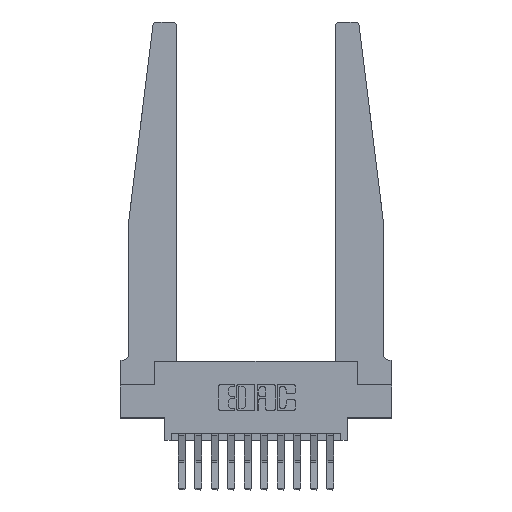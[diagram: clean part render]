
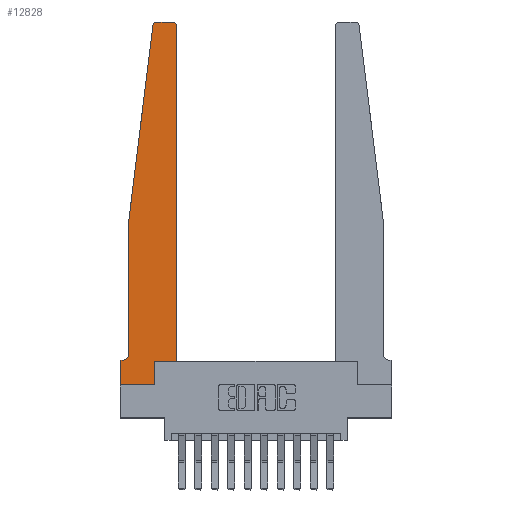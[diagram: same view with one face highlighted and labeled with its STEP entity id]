
A CAD part, top view. The second image highlights one B-rep face of the part: STEP entity #12828.
In plain terms, the highlighted planar face has unit normal (0, 0, 1).
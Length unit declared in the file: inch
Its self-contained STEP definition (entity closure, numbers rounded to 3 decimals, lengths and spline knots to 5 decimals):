
#224 = DIRECTION ( 'NONE',  ( 0., -1., 0. ) ) ;
#311 = VECTOR ( 'NONE', #13457, 39.37008 ) ;
#659 = DIRECTION ( 'NONE',  ( 1., 0., 0. ) ) ;
#852 = EDGE_LOOP ( 'NONE', ( #8478, #11043, #6783, #9050, #4390, #16160, #5548, #2327, #15677, #2943, #4963, #11494 ) ) ;
#966 = VERTEX_POINT ( 'NONE', #7093 ) ;
#1336 = DIRECTION ( 'NONE',  ( 0., 0., 1. ) ) ;
#1427 = CARTESIAN_POINT ( 'NONE',  ( 0., 0.1875, 0.37 ) ) ;
#1507 = EDGE_CURVE ( 'NONE', #2452, #4748, #9371, .T. ) ;
#1512 = VERTEX_POINT ( 'NONE', #13615 ) ;
#1540 = CARTESIAN_POINT ( 'NONE',  ( 0., 0., 0.37 ) ) ;
#1623 = AXIS2_PLACEMENT_3D ( 'NONE', #6373, #7605, #7774 ) ;
#1790 = CARTESIAN_POINT ( 'NONE',  ( 0.27653, 2.72, 0.37 ) ) ;
#2063 = VERTEX_POINT ( 'NONE', #3731 ) ;
#2226 = AXIS2_PLACEMENT_3D ( 'NONE', #1427, #1336, #9835 ) ;
#2267 = EDGE_CURVE ( 'NONE', #15915, #15272, #12274, .T. ) ;
#2270 = EDGE_CURVE ( 'NONE', #12565, #966, #16127, .T. ) ;
#2327 = ORIENTED_EDGE ( 'NONE', *, *, #6357, .T. ) ;
#2452 = VERTEX_POINT ( 'NONE', #2868 ) ;
#2659 = EDGE_CURVE ( 'NONE', #2063, #2452, #16177, .T. ) ;
#2868 = CARTESIAN_POINT ( 'NONE',  ( 0.2605, 0.18, 0.37 ) ) ;
#2943 = ORIENTED_EDGE ( 'NONE', *, *, #1507, .T. ) ;
#3179 = EDGE_CURVE ( 'NONE', #15272, #12565, #8724, .T. ) ;
#3459 = EDGE_CURVE ( 'NONE', #4748, #9136, #9968, .T. ) ;
#3561 = DIRECTION ( 'NONE',  ( 0., -1., 0. ) ) ;
#3731 = CARTESIAN_POINT ( 'NONE',  ( 0.2605, 0., 0.37 ) ) ;
#4014 = DIRECTION ( 'NONE',  ( -0.122, -0.992, 0. ) ) ;
#4219 = DIRECTION ( 'NONE',  ( -1., 0., 0. ) ) ;
#4390 = ORIENTED_EDGE ( 'NONE', *, *, #3179, .T. ) ;
#4739 = CARTESIAN_POINT ( 'NONE',  ( 0., 0., 0.37 ) ) ;
#4748 = VERTEX_POINT ( 'NONE', #13323 ) ;
#4963 = ORIENTED_EDGE ( 'NONE', *, *, #3459, .T. ) ;
#5191 = EDGE_CURVE ( 'NONE', #966, #12253, #5245, .T. ) ;
#5245 = LINE ( 'NONE', #11485, #8251 ) ;
#5548 = ORIENTED_EDGE ( 'NONE', *, *, #5191, .T. ) ;
#5680 = CIRCLE ( 'NONE', #14848, 0.03 ) ;
#5836 = DIRECTION ( 'NONE',  ( 0., 0., 1. ) ) ;
#6187 = CIRCLE ( 'NONE', #11174, 0.03 ) ;
#6225 = FACE_OUTER_BOUND ( 'NONE', #852, .T. ) ;
#6357 = EDGE_CURVE ( 'NONE', #12253, #2063, #11417, .T. ) ;
#6373 = CARTESIAN_POINT ( 'NONE',  ( 0.015, 0.2375, 0.37 ) ) ;
#6566 = DIRECTION ( 'NONE',  ( 1., 0., 0. ) ) ;
#6783 = ORIENTED_EDGE ( 'NONE', *, *, #9160, .T. ) ;
#6831 = DIRECTION ( 'NONE',  ( 0., 0., 1. ) ) ;
#7069 = CARTESIAN_POINT ( 'NONE',  ( 0.24675, 2.72367, 0.37 ) ) ;
#7093 = CARTESIAN_POINT ( 'NONE',  ( 0., 0.1875, 0.37 ) ) ;
#7200 = CARTESIAN_POINT ( 'NONE',  ( 0.065, 0.1875, 0.37 ) ) ;
#7348 = CARTESIAN_POINT ( 'NONE',  ( 0.065, 1.25, 0.37 ) ) ;
#7605 = DIRECTION ( 'NONE',  ( 0., 0., -1. ) ) ;
#7640 = EDGE_CURVE ( 'NONE', #9136, #1512, #5680, .T. ) ;
#7774 = DIRECTION ( 'NONE',  ( -1., 0., 0. ) ) ;
#8003 = VERTEX_POINT ( 'NONE', #7069 ) ;
#8140 = DIRECTION ( 'NONE',  ( 1., 0., 0. ) ) ;
#8251 = VECTOR ( 'NONE', #224, 39.37008 ) ;
#8273 = EDGE_CURVE ( 'NONE', #1512, #13807, #15478, .T. ) ;
#8478 = ORIENTED_EDGE ( 'NONE', *, *, #8273, .T. ) ;
#8719 = VECTOR ( 'NONE', #4014, 39.37008 ) ;
#8724 = CIRCLE ( 'NONE', #1623, 0.05 ) ;
#9050 = ORIENTED_EDGE ( 'NONE', *, *, #2267, .T. ) ;
#9136 = VERTEX_POINT ( 'NONE', #15598 ) ;
#9160 = EDGE_CURVE ( 'NONE', #8003, #15915, #14111, .T. ) ;
#9183 = CARTESIAN_POINT ( 'NONE',  ( 0.015, 0.1875, 0.37 ) ) ;
#9191 = CARTESIAN_POINT ( 'NONE',  ( 0.065, 1.25, 0.37 ) ) ;
#9237 = VECTOR ( 'NONE', #15960, 39.37008 ) ;
#9371 = LINE ( 'NONE', #14357, #15225 ) ;
#9597 = VECTOR ( 'NONE', #6566, 39.37008 ) ;
#9790 = VECTOR ( 'NONE', #14635, 39.37008 ) ;
#9835 = DIRECTION ( 'NONE',  ( 1., 0., 0. ) ) ;
#9968 = LINE ( 'NONE', #14882, #9790 ) ;
#10014 = VECTOR ( 'NONE', #4219, 39.37008 ) ;
#10415 = CARTESIAN_POINT ( 'NONE',  ( 0.065, 1.25, 0.37 ) ) ;
#11043 = ORIENTED_EDGE ( 'NONE', *, *, #13261, .T. ) ;
#11174 = AXIS2_PLACEMENT_3D ( 'NONE', #1790, #6831, #8140 ) ;
#11417 = LINE ( 'NONE', #1540, #9597 ) ;
#11485 = CARTESIAN_POINT ( 'NONE',  ( 0., 0., 0.37 ) ) ;
#11494 = ORIENTED_EDGE ( 'NONE', *, *, #7640, .T. ) ;
#11916 = CARTESIAN_POINT ( 'NONE',  ( 0.395, 2.72, 0.37 ) ) ;
#12253 = VERTEX_POINT ( 'NONE', #4739 ) ;
#12274 = LINE ( 'NONE', #7348, #13164 ) ;
#12538 = PLANE ( 'NONE',  #2226 ) ;
#12565 = VERTEX_POINT ( 'NONE', #9183 ) ;
#12828 = ADVANCED_FACE ( 'NONE', ( #6225 ), #12538, .T. ) ;
#13164 = VECTOR ( 'NONE', #3561, 39.37008 ) ;
#13261 = EDGE_CURVE ( 'NONE', #13807, #8003, #6187, .T. ) ;
#13323 = CARTESIAN_POINT ( 'NONE',  ( 0.425, 0.18, 0.37 ) ) ;
#13457 = DIRECTION ( 'NONE',  ( 0., 1., 0. ) ) ;
#13615 = CARTESIAN_POINT ( 'NONE',  ( 0.395, 2.75, 0.37 ) ) ;
#13807 = VERTEX_POINT ( 'NONE', #14588 ) ;
#14008 = CARTESIAN_POINT ( 'NONE',  ( 0.25, 2.75, 0.37 ) ) ;
#14111 = LINE ( 'NONE', #9191, #8719 ) ;
#14357 = CARTESIAN_POINT ( 'NONE',  ( 0.425, 0.18, 0.37 ) ) ;
#14588 = CARTESIAN_POINT ( 'NONE',  ( 0.27653, 2.75, 0.37 ) ) ;
#14635 = DIRECTION ( 'NONE',  ( 0., 1., 0. ) ) ;
#14848 = AXIS2_PLACEMENT_3D ( 'NONE', #11916, #5836, #659 ) ;
#14882 = CARTESIAN_POINT ( 'NONE',  ( 0.425, 0.18, 0.37 ) ) ;
#15225 = VECTOR ( 'NONE', #16171, 39.37008 ) ;
#15272 = VERTEX_POINT ( 'NONE', #15662 ) ;
#15478 = LINE ( 'NONE', #14008, #10014 ) ;
#15598 = CARTESIAN_POINT ( 'NONE',  ( 0.425, 2.72, 0.37 ) ) ;
#15662 = CARTESIAN_POINT ( 'NONE',  ( 0.065, 0.2375, 0.37 ) ) ;
#15677 = ORIENTED_EDGE ( 'NONE', *, *, #2659, .T. ) ;
#15915 = VERTEX_POINT ( 'NONE', #10415 ) ;
#15960 = DIRECTION ( 'NONE',  ( -1., 0., 0. ) ) ;
#16127 = LINE ( 'NONE', #7200, #9237 ) ;
#16160 = ORIENTED_EDGE ( 'NONE', *, *, #2270, .T. ) ;
#16171 = DIRECTION ( 'NONE',  ( 1., 0., 0. ) ) ;
#16177 = LINE ( 'NONE', #16250, #311 ) ;
#16250 = CARTESIAN_POINT ( 'NONE',  ( 0.2605, 0.18, 0.37 ) ) ;
